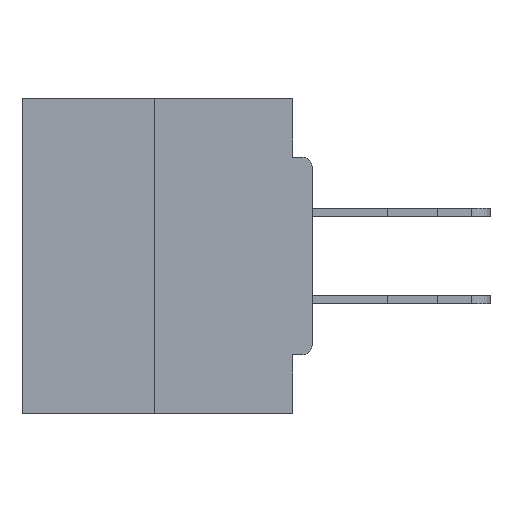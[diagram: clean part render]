
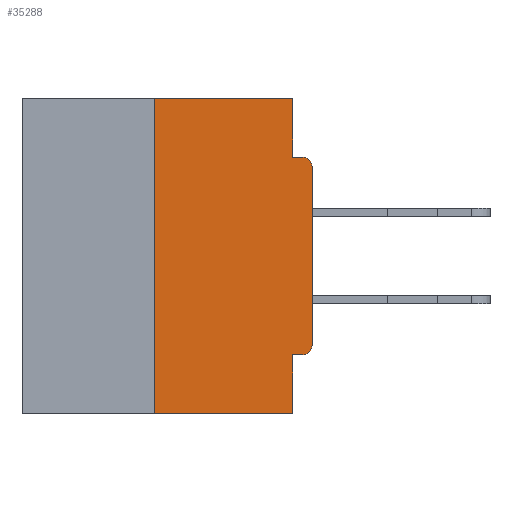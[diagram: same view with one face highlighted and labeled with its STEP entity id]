
A CAD part, left-side view. The second image highlights one B-rep face of the part: STEP entity #35288.
In plain terms, the highlighted planar face has unit normal (-1, 0, 0).
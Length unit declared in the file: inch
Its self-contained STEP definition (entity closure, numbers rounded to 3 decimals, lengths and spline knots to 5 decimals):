
#1367 = CARTESIAN_POINT ( 'NONE',  ( 0., 0.015, -0.1085 ) ) ;
#1408 = CARTESIAN_POINT ( 'NONE',  ( 0., 0., -0.3915 ) ) ;
#1449 = ORIENTED_EDGE ( 'NONE', *, *, #9425, .F. ) ;
#1927 = VERTEX_POINT ( 'NONE', #19592 ) ;
#2568 = CARTESIAN_POINT ( 'NONE',  ( 0., 0.015, -0.4065 ) ) ;
#3674 = CARTESIAN_POINT ( 'NONE',  ( 0., 0., -0.4065 ) ) ;
#3712 = VERTEX_POINT ( 'NONE', #1408 ) ;
#4171 = AXIS2_PLACEMENT_3D ( 'NONE', #29008, #15261, #29244 ) ;
#4196 = DIRECTION ( 'NONE',  ( 0., 0., -1. ) ) ;
#4305 = CARTESIAN_POINT ( 'NONE',  ( 0., 0.25, 0. ) ) ;
#4686 = VERTEX_POINT ( 'NONE', #9698 ) ;
#4979 = ORIENTED_EDGE ( 'NONE', *, *, #19865, .T. ) ;
#7751 = VERTEX_POINT ( 'NONE', #8550 ) ;
#8550 = CARTESIAN_POINT ( 'NONE',  ( 0., 0., -0.1085 ) ) ;
#9425 = EDGE_CURVE ( 'NONE', #24118, #29750, #31770, .T. ) ;
#9691 = VECTOR ( 'NONE', #15030, 39.37008 ) ;
#9698 = CARTESIAN_POINT ( 'NONE',  ( 0., 0.25, -0.5 ) ) ;
#9976 = DIRECTION ( 'NONE',  ( 0., 0., -1. ) ) ;
#10487 = CARTESIAN_POINT ( 'NONE',  ( 0., 0.46, -0.5 ) ) ;
#11765 = CIRCLE ( 'NONE', #28674, 0.015 ) ;
#11811 = AXIS2_PLACEMENT_3D ( 'NONE', #15351, #34998, #9976 ) ;
#11979 = FACE_OUTER_BOUND ( 'NONE', #21699, .T. ) ;
#12117 = DIRECTION ( 'NONE',  ( 0., -1., 0. ) ) ;
#12121 = EDGE_CURVE ( 'NONE', #29750, #1927, #35283, .T. ) ;
#12140 = DIRECTION ( 'NONE',  ( 0., 0., 1. ) ) ;
#12218 = DIRECTION ( 'NONE',  ( 0., 1., 0. ) ) ;
#13735 = VECTOR ( 'NONE', #19637, 39.37008 ) ;
#14796 = DIRECTION ( 'NONE',  ( 0., 0., -1. ) ) ;
#14906 = CARTESIAN_POINT ( 'NONE',  ( 0., 0.031, -0.5 ) ) ;
#15030 = DIRECTION ( 'NONE',  ( 0., 0., 1. ) ) ;
#15261 = DIRECTION ( 'NONE',  ( -1., 0., 0. ) ) ;
#15351 = CARTESIAN_POINT ( 'NONE',  ( 0., 0.46, 0. ) ) ;
#15965 = DIRECTION ( 'NONE',  ( 0., -1., 0. ) ) ;
#16365 = LINE ( 'NONE', #25569, #13735 ) ;
#17356 = LINE ( 'NONE', #29139, #23027 ) ;
#17602 = ORIENTED_EDGE ( 'NONE', *, *, #18829, .F. ) ;
#18388 = VERTEX_POINT ( 'NONE', #26603 ) ;
#18802 = ORIENTED_EDGE ( 'NONE', *, *, #34649, .F. ) ;
#18829 = EDGE_CURVE ( 'NONE', #4686, #35569, #32435, .T. ) ;
#19260 = ORIENTED_EDGE ( 'NONE', *, *, #27736, .F. ) ;
#19592 = CARTESIAN_POINT ( 'NONE',  ( 0., 0.031, -0.5 ) ) ;
#19637 = DIRECTION ( 'NONE',  ( 0., -1., 0. ) ) ;
#19865 = EDGE_CURVE ( 'NONE', #4686, #1927, #28459, .T. ) ;
#20053 = CIRCLE ( 'NONE', #4171, 0.015 ) ;
#20901 = DIRECTION ( 'NONE',  ( -1., 0., 0. ) ) ;
#21256 = LINE ( 'NONE', #28814, #24807 ) ;
#21358 = VECTOR ( 'NONE', #15965, 39.37008 ) ;
#21699 = EDGE_LOOP ( 'NONE', ( #30804, #17602, #4979, #24371, #1449, #35188, #29413, #27935, #19260, #18802 ) ) ;
#22059 = VERTEX_POINT ( 'NONE', #23422 ) ;
#23027 = VECTOR ( 'NONE', #12117, 39.37008 ) ;
#23422 = CARTESIAN_POINT ( 'NONE',  ( 0., 0.015, -0.0935 ) ) ;
#24027 = PLANE ( 'NONE',  #11811 ) ;
#24118 = VERTEX_POINT ( 'NONE', #2568 ) ;
#24324 = EDGE_CURVE ( 'NONE', #24118, #3712, #20053, .T. ) ;
#24371 = ORIENTED_EDGE ( 'NONE', *, *, #12121, .F. ) ;
#24807 = VECTOR ( 'NONE', #12140, 39.37008 ) ;
#25569 = CARTESIAN_POINT ( 'NONE',  ( 0., 0.46, 0. ) ) ;
#25832 = CARTESIAN_POINT ( 'NONE',  ( 0., 0.031, -0.4065 ) ) ;
#26366 = EDGE_CURVE ( 'NONE', #7751, #22059, #11765, .T. ) ;
#26603 = CARTESIAN_POINT ( 'NONE',  ( 0., 0.031, -0.0935 ) ) ;
#26964 = VECTOR ( 'NONE', #12218, 39.37008 ) ;
#27548 = EDGE_CURVE ( 'NONE', #3712, #7751, #21256, .T. ) ;
#27736 = EDGE_CURVE ( 'NONE', #18388, #22059, #17356, .T. ) ;
#27935 = ORIENTED_EDGE ( 'NONE', *, *, #26366, .T. ) ;
#28459 = LINE ( 'NONE', #10487, #21358 ) ;
#28674 = AXIS2_PLACEMENT_3D ( 'NONE', #1367, #20901, #4196 ) ;
#28814 = CARTESIAN_POINT ( 'NONE',  ( 0., 0., 0. ) ) ;
#29008 = CARTESIAN_POINT ( 'NONE',  ( 0., 0.015, -0.3915 ) ) ;
#29139 = CARTESIAN_POINT ( 'NONE',  ( 0., 0., -0.0935 ) ) ;
#29244 = DIRECTION ( 'NONE',  ( 0., 0., -1. ) ) ;
#29413 = ORIENTED_EDGE ( 'NONE', *, *, #27548, .T. ) ;
#29750 = VERTEX_POINT ( 'NONE', #25832 ) ;
#30804 = ORIENTED_EDGE ( 'NONE', *, *, #35028, .F. ) ;
#31270 = CARTESIAN_POINT ( 'NONE',  ( 0., 0.25, 0. ) ) ;
#31759 = VECTOR ( 'NONE', #31973, 39.37008 ) ;
#31770 = LINE ( 'NONE', #3674, #26964 ) ;
#31973 = DIRECTION ( 'NONE',  ( 0., 0., -1. ) ) ;
#32179 = LINE ( 'NONE', #34588, #31759 ) ;
#32435 = LINE ( 'NONE', #4305, #9691 ) ;
#33486 = CARTESIAN_POINT ( 'NONE',  ( 0., 0.031, 0. ) ) ;
#34330 = VERTEX_POINT ( 'NONE', #33486 ) ;
#34393 = VECTOR ( 'NONE', #14796, 39.37008 ) ;
#34588 = CARTESIAN_POINT ( 'NONE',  ( 0., 0.031, 0. ) ) ;
#34649 = EDGE_CURVE ( 'NONE', #34330, #18388, #32179, .T. ) ;
#34998 = DIRECTION ( 'NONE',  ( 1., 0., 0. ) ) ;
#35028 = EDGE_CURVE ( 'NONE', #35569, #34330, #16365, .T. ) ;
#35188 = ORIENTED_EDGE ( 'NONE', *, *, #24324, .T. ) ;
#35283 = LINE ( 'NONE', #14906, #34393 ) ;
#35288 = ADVANCED_FACE ( 'NONE', ( #11979 ), #24027, .F. ) ;
#35569 = VERTEX_POINT ( 'NONE', #31270 ) ;
